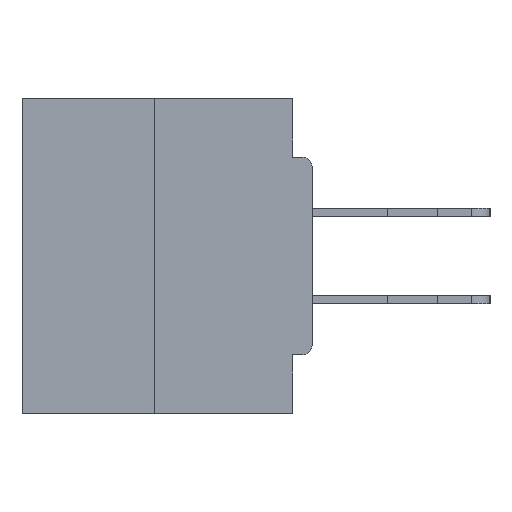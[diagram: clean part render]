
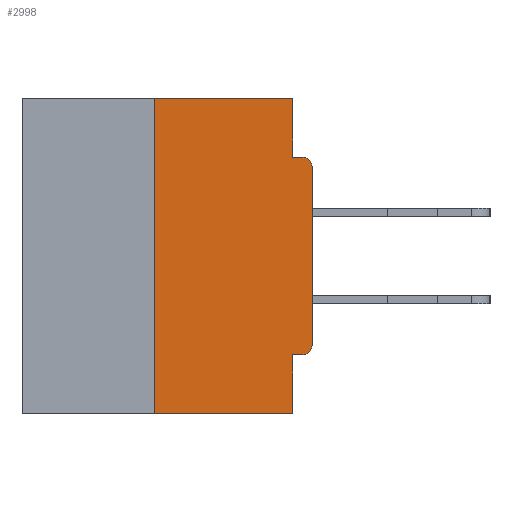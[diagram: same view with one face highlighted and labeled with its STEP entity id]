
A CAD part, left-side view. The second image highlights one B-rep face of the part: STEP entity #2998.
In plain terms, the highlighted planar face has unit normal (-1, 0, 0).
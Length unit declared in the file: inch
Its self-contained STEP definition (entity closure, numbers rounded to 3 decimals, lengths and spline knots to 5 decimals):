
#61 = CARTESIAN_POINT ( 'NONE',  ( 0., 0.031, -0.0935 ) ) ;
#198 = ORIENTED_EDGE ( 'NONE', *, *, #21381, .F. ) ;
#1910 = ORIENTED_EDGE ( 'NONE', *, *, #21541, .T. ) ;
#2139 = LINE ( 'NONE', #15240, #13879 ) ;
#2202 = CARTESIAN_POINT ( 'NONE',  ( 0., 0., -0.3915 ) ) ;
#2998 = ADVANCED_FACE ( 'NONE', ( #33886 ), #28678, .F. ) ;
#2999 = VERTEX_POINT ( 'NONE', #2202 ) ;
#4221 = VERTEX_POINT ( 'NONE', #5402 ) ;
#4818 = VECTOR ( 'NONE', #24513, 39.37008 ) ;
#5402 = CARTESIAN_POINT ( 'NONE',  ( 0., 0.031, 0. ) ) ;
#5867 = LINE ( 'NONE', #21909, #4818 ) ;
#5900 = EDGE_CURVE ( 'NONE', #14894, #4221, #13910, .T. ) ;
#7482 = AXIS2_PLACEMENT_3D ( 'NONE', #19516, #25424, #14452 ) ;
#7999 = EDGE_CURVE ( 'NONE', #21835, #26868, #17505, .T. ) ;
#8887 = DIRECTION ( 'NONE',  ( 0., 0., 1. ) ) ;
#9218 = CARTESIAN_POINT ( 'NONE',  ( 0., 0.031, -0.5 ) ) ;
#9480 = CARTESIAN_POINT ( 'NONE',  ( 0., 0., -0.0935 ) ) ;
#9658 = DIRECTION ( 'NONE',  ( 0., -1., 0. ) ) ;
#10159 = VERTEX_POINT ( 'NONE', #26664 ) ;
#10804 = VERTEX_POINT ( 'NONE', #31055 ) ;
#10942 = EDGE_CURVE ( 'NONE', #2999, #28509, #13145, .T. ) ;
#11434 = ORIENTED_EDGE ( 'NONE', *, *, #7999, .F. ) ;
#11823 = CARTESIAN_POINT ( 'NONE',  ( 0., 0.015, -0.4065 ) ) ;
#11928 = AXIS2_PLACEMENT_3D ( 'NONE', #31629, #26433, #31282 ) ;
#11966 = EDGE_CURVE ( 'NONE', #4221, #21835, #2139, .T. ) ;
#12262 = DIRECTION ( 'NONE',  ( 0., 0., -1. ) ) ;
#12431 = VECTOR ( 'NONE', #26135, 39.37008 ) ;
#12549 = LINE ( 'NONE', #25446, #12431 ) ;
#13145 = LINE ( 'NONE', #28792, #23357 ) ;
#13666 = CARTESIAN_POINT ( 'NONE',  ( 0., 0.015, -0.0935 ) ) ;
#13879 = VECTOR ( 'NONE', #12262, 39.37008 ) ;
#13910 = LINE ( 'NONE', #18959, #21824 ) ;
#14253 = DIRECTION ( 'NONE',  ( 0., 0., -1. ) ) ;
#14452 = DIRECTION ( 'NONE',  ( 0., 0., -1. ) ) ;
#14894 = VERTEX_POINT ( 'NONE', #32072 ) ;
#14914 = ORIENTED_EDGE ( 'NONE', *, *, #10942, .T. ) ;
#15240 = CARTESIAN_POINT ( 'NONE',  ( 0., 0.031, 0. ) ) ;
#15861 = EDGE_CURVE ( 'NONE', #31970, #10159, #33052, .T. ) ;
#16875 = ORIENTED_EDGE ( 'NONE', *, *, #18619, .F. ) ;
#17033 = DIRECTION ( 'NONE',  ( -1., 0., 0. ) ) ;
#17505 = LINE ( 'NONE', #9480, #30495 ) ;
#17687 = CARTESIAN_POINT ( 'NONE',  ( 0., 0.031, -0.4065 ) ) ;
#17743 = ORIENTED_EDGE ( 'NONE', *, *, #15861, .F. ) ;
#18145 = ORIENTED_EDGE ( 'NONE', *, *, #27863, .T. ) ;
#18559 = CARTESIAN_POINT ( 'NONE',  ( 0., 0., -0.1085 ) ) ;
#18619 = EDGE_CURVE ( 'NONE', #22402, #31970, #5867, .T. ) ;
#18959 = CARTESIAN_POINT ( 'NONE',  ( 0., 0.46, 0. ) ) ;
#19516 = CARTESIAN_POINT ( 'NONE',  ( 0., 0.015, -0.3915 ) ) ;
#21381 = EDGE_CURVE ( 'NONE', #10804, #14894, #24931, .T. ) ;
#21541 = EDGE_CURVE ( 'NONE', #10804, #10159, #12549, .T. ) ;
#21824 = VECTOR ( 'NONE', #24533, 39.37008 ) ;
#21835 = VERTEX_POINT ( 'NONE', #61 ) ;
#21909 = CARTESIAN_POINT ( 'NONE',  ( 0., 0., -0.4065 ) ) ;
#21967 = ORIENTED_EDGE ( 'NONE', *, *, #27479, .T. ) ;
#22402 = VERTEX_POINT ( 'NONE', #11823 ) ;
#22440 = CARTESIAN_POINT ( 'NONE',  ( 0., 0.015, -0.1085 ) ) ;
#23020 = ORIENTED_EDGE ( 'NONE', *, *, #11966, .F. ) ;
#23357 = VECTOR ( 'NONE', #23782, 39.37008 ) ;
#23726 = EDGE_LOOP ( 'NONE', ( #27872, #198, #1910, #17743, #16875, #21967, #14914, #18145, #11434, #23020 ) ) ;
#23782 = DIRECTION ( 'NONE',  ( 0., 0., 1. ) ) ;
#24213 = CIRCLE ( 'NONE', #25874, 0.015 ) ;
#24513 = DIRECTION ( 'NONE',  ( 0., 1., 0. ) ) ;
#24533 = DIRECTION ( 'NONE',  ( 0., -1., 0. ) ) ;
#24931 = LINE ( 'NONE', #32732, #27995 ) ;
#25424 = DIRECTION ( 'NONE',  ( -1., 0., 0. ) ) ;
#25446 = CARTESIAN_POINT ( 'NONE',  ( 0., 0.46, -0.5 ) ) ;
#25874 = AXIS2_PLACEMENT_3D ( 'NONE', #22440, #17033, #14253 ) ;
#26135 = DIRECTION ( 'NONE',  ( 0., -1., 0. ) ) ;
#26433 = DIRECTION ( 'NONE',  ( 1., 0., 0. ) ) ;
#26664 = CARTESIAN_POINT ( 'NONE',  ( 0., 0.031, -0.5 ) ) ;
#26868 = VERTEX_POINT ( 'NONE', #13666 ) ;
#27479 = EDGE_CURVE ( 'NONE', #22402, #2999, #33027, .T. ) ;
#27863 = EDGE_CURVE ( 'NONE', #28509, #26868, #24213, .T. ) ;
#27872 = ORIENTED_EDGE ( 'NONE', *, *, #5900, .F. ) ;
#27995 = VECTOR ( 'NONE', #8887, 39.37008 ) ;
#28509 = VERTEX_POINT ( 'NONE', #18559 ) ;
#28678 = PLANE ( 'NONE',  #11928 ) ;
#28792 = CARTESIAN_POINT ( 'NONE',  ( 0., 0., 0. ) ) ;
#30445 = DIRECTION ( 'NONE',  ( 0., 0., -1. ) ) ;
#30495 = VECTOR ( 'NONE', #9658, 39.37008 ) ;
#31055 = CARTESIAN_POINT ( 'NONE',  ( 0., 0.25, -0.5 ) ) ;
#31282 = DIRECTION ( 'NONE',  ( 0., 0., -1. ) ) ;
#31629 = CARTESIAN_POINT ( 'NONE',  ( 0., 0.46, 0. ) ) ;
#31970 = VERTEX_POINT ( 'NONE', #17687 ) ;
#32072 = CARTESIAN_POINT ( 'NONE',  ( 0., 0.25, 0. ) ) ;
#32732 = CARTESIAN_POINT ( 'NONE',  ( 0., 0.25, 0. ) ) ;
#33027 = CIRCLE ( 'NONE', #7482, 0.015 ) ;
#33052 = LINE ( 'NONE', #9218, #33542 ) ;
#33542 = VECTOR ( 'NONE', #30445, 39.37008 ) ;
#33886 = FACE_OUTER_BOUND ( 'NONE', #23726, .T. ) ;
